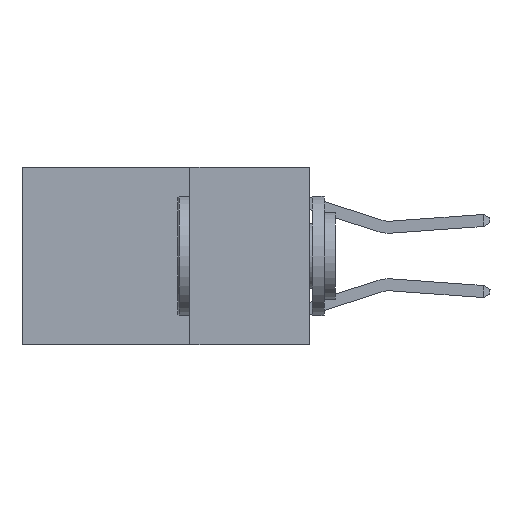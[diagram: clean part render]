
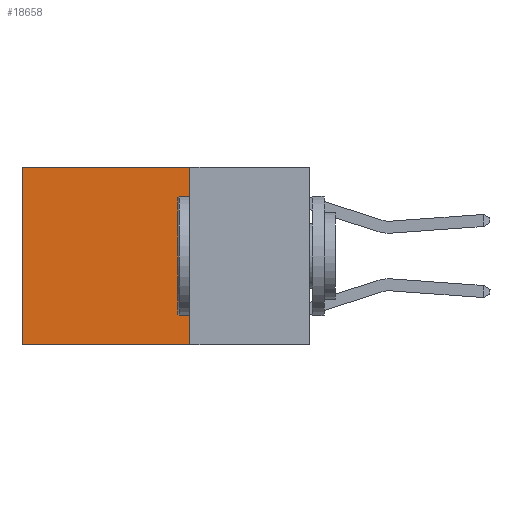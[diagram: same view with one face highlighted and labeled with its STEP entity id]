
A CAD part, left-side view. The second image highlights one B-rep face of the part: STEP entity #18658.
In plain terms, the highlighted planar face has unit normal (-1, 0, 0).
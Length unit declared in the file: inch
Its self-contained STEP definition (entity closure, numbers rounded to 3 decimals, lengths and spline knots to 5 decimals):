
#62 = ORIENTED_EDGE ( 'NONE', *, *, #10833, .F. ) ;
#161 = ORIENTED_EDGE ( 'NONE', *, *, #22440, .F. ) ;
#1770 = DIRECTION ( 'NONE',  ( 1., 0., 0. ) ) ;
#3335 = DIRECTION ( 'NONE',  ( 0., 0., -1. ) ) ;
#3469 = VECTOR ( 'NONE', #9492, 39.37008 ) ;
#3489 = LINE ( 'NONE', #29315, #16952 ) ;
#3858 = EDGE_LOOP ( 'NONE', ( #13379, #62, #161, #4463 ) ) ;
#4368 = VERTEX_POINT ( 'NONE', #24823 ) ;
#4463 = ORIENTED_EDGE ( 'NONE', *, *, #21775, .T. ) ;
#5527 = AXIS2_PLACEMENT_3D ( 'NONE', #27823, #1770, #18476 ) ;
#5907 = DIRECTION ( 'NONE',  ( 0., 1., 0. ) ) ;
#6985 = CARTESIAN_POINT ( 'NONE',  ( 0.2625, 0.25, -0.37 ) ) ;
#9492 = DIRECTION ( 'NONE',  ( 0., 1., 0. ) ) ;
#9620 = LINE ( 'NONE', #20139, #27679 ) ;
#10833 = EDGE_CURVE ( 'NONE', #4368, #29424, #22491, .T. ) ;
#11245 = PLANE ( 'NONE',  #5527 ) ;
#13379 = ORIENTED_EDGE ( 'NONE', *, *, #16471, .T. ) ;
#14138 = VERTEX_POINT ( 'NONE', #21581 ) ;
#15256 = DIRECTION ( 'NONE',  ( 0., 0., -1. ) ) ;
#15588 = CARTESIAN_POINT ( 'NONE',  ( 0.2625, 0.6, 0. ) ) ;
#16471 = EDGE_CURVE ( 'NONE', #25387, #29424, #21481, .T. ) ;
#16952 = VECTOR ( 'NONE', #15256, 39.37008 ) ;
#18476 = DIRECTION ( 'NONE',  ( 0., 0., -1. ) ) ;
#18658 = ADVANCED_FACE ( 'NONE', ( #28266 ), #11245, .F. ) ;
#20139 = CARTESIAN_POINT ( 'NONE',  ( 0.2625, 0.25, 0. ) ) ;
#21481 = LINE ( 'NONE', #24658, #25499 ) ;
#21581 = CARTESIAN_POINT ( 'NONE',  ( 0.2625, 0.25, 0. ) ) ;
#21775 = EDGE_CURVE ( 'NONE', #14138, #25387, #9620, .T. ) ;
#22440 = EDGE_CURVE ( 'NONE', #14138, #4368, #3489, .T. ) ;
#22491 = LINE ( 'NONE', #6985, #3469 ) ;
#24658 = CARTESIAN_POINT ( 'NONE',  ( 0.2625, 0.6, 0. ) ) ;
#24823 = CARTESIAN_POINT ( 'NONE',  ( 0.2625, 0.25, -0.37 ) ) ;
#25387 = VERTEX_POINT ( 'NONE', #15588 ) ;
#25499 = VECTOR ( 'NONE', #3335, 39.37008 ) ;
#25796 = CARTESIAN_POINT ( 'NONE',  ( 0.2625, 0.6, -0.37 ) ) ;
#27679 = VECTOR ( 'NONE', #5907, 39.37008 ) ;
#27823 = CARTESIAN_POINT ( 'NONE',  ( 0.2625, 0.25, 0. ) ) ;
#28266 = FACE_OUTER_BOUND ( 'NONE', #3858, .T. ) ;
#29315 = CARTESIAN_POINT ( 'NONE',  ( 0.2625, 0.25, 0. ) ) ;
#29424 = VERTEX_POINT ( 'NONE', #25796 ) ;
